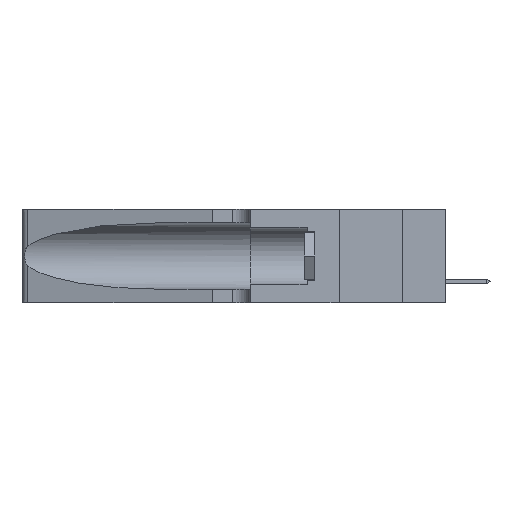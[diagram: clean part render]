
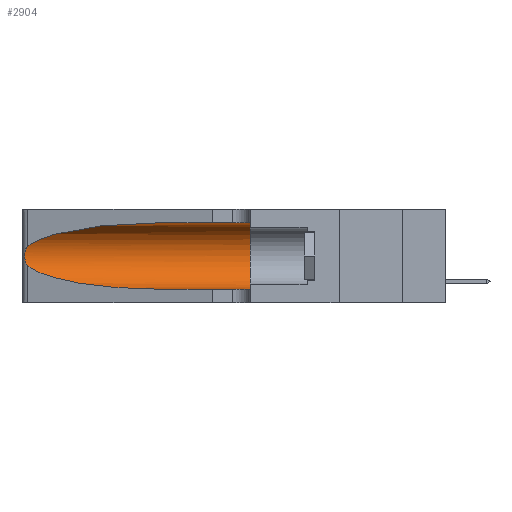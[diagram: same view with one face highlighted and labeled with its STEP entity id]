
A CAD part, left-side view. The second image highlights one B-rep face of the part: STEP entity #2904.
In plain terms, the highlighted cylindrical face has radius 3.308 mm (diameter 6.617 mm), a partial arc.
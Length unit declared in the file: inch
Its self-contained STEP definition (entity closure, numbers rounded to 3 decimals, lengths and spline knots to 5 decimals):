
#1565 = CARTESIAN_POINT ( 'NONE',  ( 0.1305, 0.72297, 0.05475 ) ) ;
#1806 =( BOUNDED_CURVE ( )  B_SPLINE_CURVE ( 3, ( #15922, #7930, #4849, #1565 ),
 .UNSPECIFIED., .F., .F. ) 
 B_SPLINE_CURVE_WITH_KNOTS ( ( 4, 4 ),
 ( 3.44316, 4.71239 ),
 .UNSPECIFIED. ) 
 CURVE ( )  GEOMETRIC_REPRESENTATION_ITEM ( )  RATIONAL_B_SPLINE_CURVE ( ( 1., 0.87, 0.87, 1. ) ) 
 REPRESENTATION_ITEM ( '' )  );
#1925 = DIRECTION ( 'NONE',  ( 0., -1., 0. ) ) ;
#2475 = CARTESIAN_POINT ( 'NONE',  ( 0.1305, 0.72297, 0.31525 ) ) ;
#2904 = ADVANCED_FACE ( 'NONE', ( #14720 ), #3660, .F. ) ;
#3432 = VERTEX_POINT ( 'NONE', #2475 ) ;
#3660 = CYLINDRICAL_SURFACE ( 'NONE', #4043, 0.13025 ) ;
#4043 = AXIS2_PLACEMENT_3D ( 'NONE', #17616, #11416, #11757 ) ;
#4239 = ORIENTED_EDGE ( 'NONE', *, *, #12295, .F. ) ;
#4815 = VECTOR ( 'NONE', #1925, 39.37008 ) ;
#4849 = CARTESIAN_POINT ( 'NONE',  ( 0.18966, 0.96281, 0.05475 ) ) ;
#5292 = LINE ( 'NONE', #6443, #4815 ) ;
#5304 = CARTESIAN_POINT ( 'NONE',  ( 0.1305, 0.35, 0.05475 ) ) ;
#5963 = CARTESIAN_POINT ( 'NONE',  ( 0.1305, 1.61858, 0.05475 ) ) ;
#6143 = CARTESIAN_POINT ( 'NONE',  ( 0.18966, 0.96281, 0.31525 ) ) ;
#6443 = CARTESIAN_POINT ( 'NONE',  ( 0.1305, 1.61858, 0.31525 ) ) ;
#6963 = VECTOR ( 'NONE', #20169, 39.37008 ) ;
#7186 = CARTESIAN_POINT ( 'NONE',  ( 0.25789, 1.23486, 0.15765 ) ) ;
#7930 = CARTESIAN_POINT ( 'NONE',  ( 0.2373, 1.15595, 0.08982 ) ) ;
#9192 = ORIENTED_EDGE ( 'NONE', *, *, #12527, .F. ) ;
#9327 = CARTESIAN_POINT ( 'NONE',  ( 0.25555, 1.22994, 0.2215 ) ) ;
#9670 = CARTESIAN_POINT ( 'NONE',  ( 0.25854, 1.2359, 0.20912 ) ) ;
#9834 = EDGE_CURVE ( 'NONE', #3432, #18851, #20234, .T. ) ;
#10360 = DIRECTION ( 'NONE',  ( 0., 1., 0. ) ) ;
#10385 = B_SPLINE_CURVE_WITH_KNOTS ( 'NONE', 3,
 ( #15648, #9327, #15444, #19018, #9670, #14385, #11085, #16194, #17857, #10608, #7186, #11985, #16587, #16782 ),
 .UNSPECIFIED., .F., .F.,
 ( 4, 2, 2, 2, 2, 2, 4 ),
 ( 0., 0.00027, 0.00053, 0.00107, 0.0016, 0.00187, 0.00214 ),
 .UNSPECIFIED. ) ;
#10497 = CARTESIAN_POINT ( 'NONE',  ( 0.25487, 1.22718, 0.14631 ) ) ;
#10608 = CARTESIAN_POINT ( 'NONE',  ( 0.25856, 1.23593, 0.16098 ) ) ;
#10870 = CARTESIAN_POINT ( 'NONE',  ( 0.25487, 1.22718, 0.22369 ) ) ;
#11085 = CARTESIAN_POINT ( 'NONE',  ( 0.26075, 1.23896, 0.19203 ) ) ;
#11217 = LINE ( 'NONE', #5963, #6963 ) ;
#11416 = DIRECTION ( 'NONE',  ( 0., -1., 0. ) ) ;
#11757 = DIRECTION ( 'NONE',  ( 0., 0., -1. ) ) ;
#11889 = AXIS2_PLACEMENT_3D ( 'NONE', #11954, #10360, #16983 ) ;
#11954 = CARTESIAN_POINT ( 'NONE',  ( 0.1305, 0.35, 0.185 ) ) ;
#11985 = CARTESIAN_POINT ( 'NONE',  ( 0.25639, 1.23186, 0.15144 ) ) ;
#12295 = EDGE_CURVE ( 'NONE', #16650, #16908, #15414, .T. ) ;
#12527 = EDGE_CURVE ( 'NONE', #3432, #16650, #5292, .T. ) ;
#13427 = EDGE_CURVE ( 'NONE', #17098, #14060, #1806, .T. ) ;
#13518 = CARTESIAN_POINT ( 'NONE',  ( 0.1305, 0.35, 0.31525 ) ) ;
#14060 = VERTEX_POINT ( 'NONE', #19539 ) ;
#14385 = CARTESIAN_POINT ( 'NONE',  ( 0.26018, 1.23835, 0.19895 ) ) ;
#14720 = FACE_OUTER_BOUND ( 'NONE', #16157, .T. ) ;
#15290 = ORIENTED_EDGE ( 'NONE', *, *, #9834, .T. ) ;
#15414 = CIRCLE ( 'NONE', #11889, 0.13025 ) ;
#15444 = CARTESIAN_POINT ( 'NONE',  ( 0.25639, 1.23184, 0.21858 ) ) ;
#15509 = CARTESIAN_POINT ( 'NONE',  ( 0.1305, 0.72297, 0.31525 ) ) ;
#15648 = CARTESIAN_POINT ( 'NONE',  ( 0.25487, 1.22718, 0.22369 ) ) ;
#15922 = CARTESIAN_POINT ( 'NONE',  ( 0.25487, 1.22718, 0.14631 ) ) ;
#16157 = EDGE_LOOP ( 'NONE', ( #15290, #17170, #16520, #18850, #4239, #9192 ) ) ;
#16194 = CARTESIAN_POINT ( 'NONE',  ( 0.26075, 1.23896, 0.178 ) ) ;
#16520 = ORIENTED_EDGE ( 'NONE', *, *, #13427, .T. ) ;
#16587 = CARTESIAN_POINT ( 'NONE',  ( 0.25555, 1.22993, 0.14849 ) ) ;
#16650 = VERTEX_POINT ( 'NONE', #13518 ) ;
#16724 = EDGE_CURVE ( 'NONE', #18851, #17098, #10385, .T. ) ;
#16782 = CARTESIAN_POINT ( 'NONE',  ( 0.25487, 1.22718, 0.14631 ) ) ;
#16908 = VERTEX_POINT ( 'NONE', #5304 ) ;
#16983 = DIRECTION ( 'NONE',  ( 0., 0., 1. ) ) ;
#17098 = VERTEX_POINT ( 'NONE', #10497 ) ;
#17170 = ORIENTED_EDGE ( 'NONE', *, *, #16724, .T. ) ;
#17354 = CARTESIAN_POINT ( 'NONE',  ( 0.25487, 1.22718, 0.22369 ) ) ;
#17616 = CARTESIAN_POINT ( 'NONE',  ( 0.1305, 1.61858, 0.185 ) ) ;
#17857 = CARTESIAN_POINT ( 'NONE',  ( 0.26017, 1.23833, 0.17102 ) ) ;
#18850 = ORIENTED_EDGE ( 'NONE', *, *, #19226, .T. ) ;
#18851 = VERTEX_POINT ( 'NONE', #17354 ) ;
#19018 = CARTESIAN_POINT ( 'NONE',  ( 0.25787, 1.23484, 0.2124 ) ) ;
#19226 = EDGE_CURVE ( 'NONE', #14060, #16908, #11217, .T. ) ;
#19539 = CARTESIAN_POINT ( 'NONE',  ( 0.1305, 0.72297, 0.05475 ) ) ;
#20144 = CARTESIAN_POINT ( 'NONE',  ( 0.2373, 1.15595, 0.28018 ) ) ;
#20169 = DIRECTION ( 'NONE',  ( 0., -1., 0. ) ) ;
#20234 =( BOUNDED_CURVE ( )  B_SPLINE_CURVE ( 3, ( #15509, #6143, #20144, #10870 ),
 .UNSPECIFIED., .F., .F. ) 
 B_SPLINE_CURVE_WITH_KNOTS ( ( 4, 4 ),
 ( 1.5708, 2.84003 ),
 .UNSPECIFIED. ) 
 CURVE ( )  GEOMETRIC_REPRESENTATION_ITEM ( )  RATIONAL_B_SPLINE_CURVE ( ( 1., 0.87, 0.87, 1. ) ) 
 REPRESENTATION_ITEM ( '' )  );
